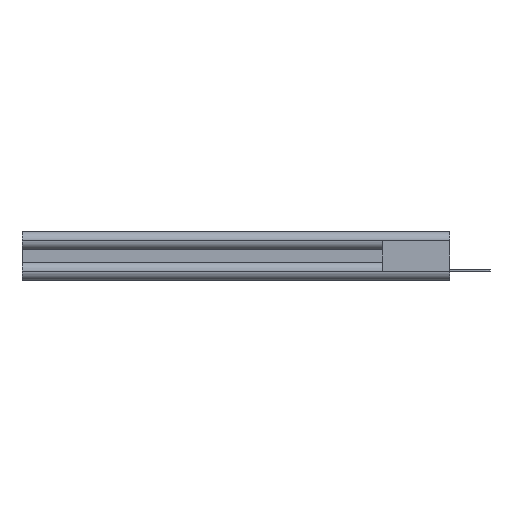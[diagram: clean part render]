
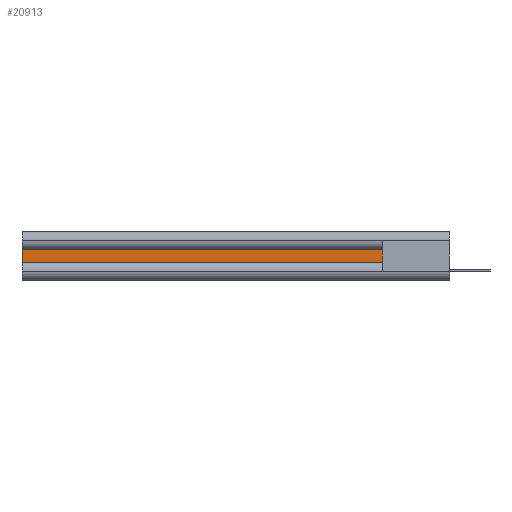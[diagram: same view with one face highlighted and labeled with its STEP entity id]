
A CAD part, left-side view. The second image highlights one B-rep face of the part: STEP entity #20913.
In plain terms, the highlighted planar face has unit normal (-1, 0, 0).
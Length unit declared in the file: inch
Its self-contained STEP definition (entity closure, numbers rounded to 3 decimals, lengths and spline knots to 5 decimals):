
#804 = CARTESIAN_POINT ( 'NONE',  ( 0.044, 0.473, -0.0465 ) ) ;
#1672 = VERTEX_POINT ( 'NONE', #9865 ) ;
#1934 = CARTESIAN_POINT ( 'NONE',  ( 0.044, 0.37012, 0.0465 ) ) ;
#3053 = VECTOR ( 'NONE', #18930, 39.37008 ) ;
#3113 = DIRECTION ( 'NONE',  ( 0., 0., -1. ) ) ;
#3294 = LINE ( 'NONE', #1934, #11816 ) ;
#3368 = ORIENTED_EDGE ( 'NONE', *, *, #10124, .F. ) ;
#3600 = DIRECTION ( 'NONE',  ( 0., 1., 0. ) ) ;
#3670 = VECTOR ( 'NONE', #10347, 39.37008 ) ;
#4075 = ORIENTED_EDGE ( 'NONE', *, *, #7650, .T. ) ;
#4144 = AXIS2_PLACEMENT_3D ( 'NONE', #4734, #13293, #3113 ) ;
#4734 = CARTESIAN_POINT ( 'NONE',  ( 0.044, 0.37012, -0.0465 ) ) ;
#5154 = EDGE_LOOP ( 'NONE', ( #4075, #16385, #3368, #7852 ) ) ;
#6046 = VERTEX_POINT ( 'NONE', #12381 ) ;
#7273 = VERTEX_POINT ( 'NONE', #17665 ) ;
#7275 = DIRECTION ( 'NONE',  ( 0., 0., -1. ) ) ;
#7572 = LINE ( 'NONE', #12188, #3053 ) ;
#7650 = EDGE_CURVE ( 'NONE', #7273, #6046, #3294, .T. ) ;
#7852 = ORIENTED_EDGE ( 'NONE', *, *, #12761, .F. ) ;
#8635 = CARTESIAN_POINT ( 'NONE',  ( 0.044, 0.37012, -0.0465 ) ) ;
#9865 = CARTESIAN_POINT ( 'NONE',  ( 0.044, 3., -0.0465 ) ) ;
#10124 = EDGE_CURVE ( 'NONE', #12276, #1672, #12725, .T. ) ;
#10347 = DIRECTION ( 'NONE',  ( 0., 1., 0. ) ) ;
#11035 = VECTOR ( 'NONE', #7275, 39.37008 ) ;
#11816 = VECTOR ( 'NONE', #3600, 39.37008 ) ;
#12188 = CARTESIAN_POINT ( 'NONE',  ( 0.044, 0.473, -0.0465 ) ) ;
#12276 = VERTEX_POINT ( 'NONE', #804 ) ;
#12381 = CARTESIAN_POINT ( 'NONE',  ( 0.044, 3., 0.0465 ) ) ;
#12725 = LINE ( 'NONE', #8635, #3670 ) ;
#12761 = EDGE_CURVE ( 'NONE', #7273, #12276, #7572, .T. ) ;
#12801 = EDGE_CURVE ( 'NONE', #6046, #1672, #15492, .T. ) ;
#13293 = DIRECTION ( 'NONE',  ( 1., 0., 0. ) ) ;
#14019 = CARTESIAN_POINT ( 'NONE',  ( 0.044, 3., -0.0465 ) ) ;
#15492 = LINE ( 'NONE', #14019, #11035 ) ;
#16385 = ORIENTED_EDGE ( 'NONE', *, *, #12801, .T. ) ;
#17665 = CARTESIAN_POINT ( 'NONE',  ( 0.044, 0.473, 0.0465 ) ) ;
#18259 = PLANE ( 'NONE',  #4144 ) ;
#18930 = DIRECTION ( 'NONE',  ( 0., 0., -1. ) ) ;
#20674 = FACE_OUTER_BOUND ( 'NONE', #5154, .T. ) ;
#20913 = ADVANCED_FACE ( 'NONE', ( #20674 ), #18259, .F. ) ;
